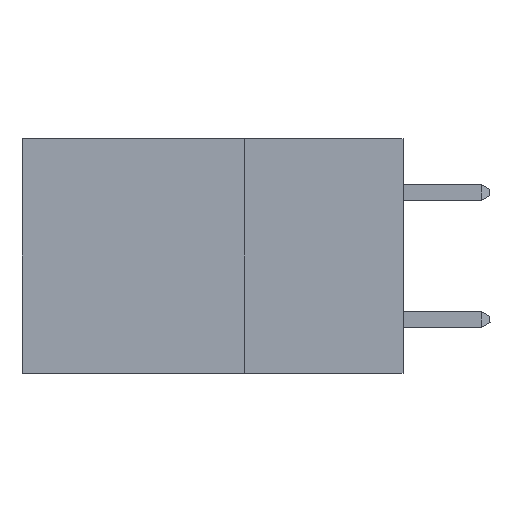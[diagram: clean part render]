
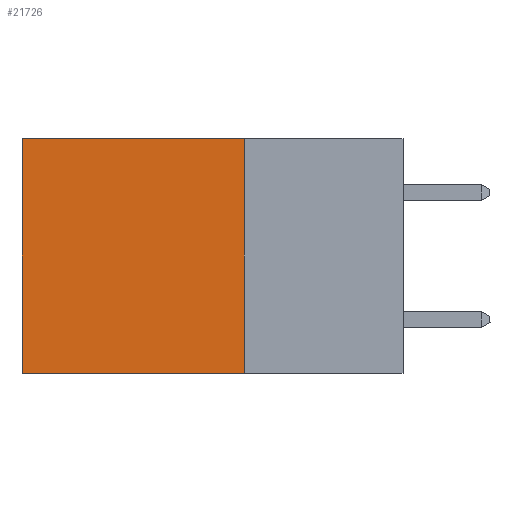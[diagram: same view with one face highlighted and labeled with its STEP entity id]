
A CAD part, left-side view. The second image highlights one B-rep face of the part: STEP entity #21726.
In plain terms, the highlighted planar face has unit normal (-1, 0, 0).
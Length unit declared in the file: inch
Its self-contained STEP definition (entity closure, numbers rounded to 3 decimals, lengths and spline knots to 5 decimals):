
#52 = PLANE ( 'NONE',  #2230 ) ;
#2230 = AXIS2_PLACEMENT_3D ( 'NONE', #5480, #8136, #5143 ) ;
#2328 = DIRECTION ( 'NONE',  ( 0., 0., -1. ) ) ;
#2880 = VERTEX_POINT ( 'NONE', #23018 ) ;
#3109 = CARTESIAN_POINT ( 'NONE',  ( 0.2875, 0.25, -0.37 ) ) ;
#4250 = EDGE_CURVE ( 'NONE', #25213, #13883, #14950, .T. ) ;
#5143 = DIRECTION ( 'NONE',  ( 0., 0., -1. ) ) ;
#5480 = CARTESIAN_POINT ( 'NONE',  ( 0.2875, 0.25, 0. ) ) ;
#6723 = VECTOR ( 'NONE', #2328, 39.37008 ) ;
#7089 = CARTESIAN_POINT ( 'NONE',  ( 0.2875, 0.6, 0. ) ) ;
#8136 = DIRECTION ( 'NONE',  ( 1., 0., 0. ) ) ;
#8657 = CARTESIAN_POINT ( 'NONE',  ( 0.2875, 0.25, -0.37 ) ) ;
#12999 = LINE ( 'NONE', #7089, #6723 ) ;
#13883 = VERTEX_POINT ( 'NONE', #3109 ) ;
#14950 = LINE ( 'NONE', #15391, #26973 ) ;
#15224 = LINE ( 'NONE', #8657, #28020 ) ;
#15391 = CARTESIAN_POINT ( 'NONE',  ( 0.2875, 0.25, 0. ) ) ;
#15589 = FACE_OUTER_BOUND ( 'NONE', #30320, .T. ) ;
#17934 = DIRECTION ( 'NONE',  ( 0., 0., -1. ) ) ;
#18695 = LINE ( 'NONE', #27584, #28721 ) ;
#19436 = CARTESIAN_POINT ( 'NONE',  ( 0.2875, 0.25, 0. ) ) ;
#21438 = EDGE_CURVE ( 'NONE', #13883, #29288, #15224, .T. ) ;
#21726 = ADVANCED_FACE ( 'NONE', ( #15589 ), #52, .F. ) ;
#22998 = ORIENTED_EDGE ( 'NONE', *, *, #4250, .F. ) ;
#23018 = CARTESIAN_POINT ( 'NONE',  ( 0.2875, 0.6, 0. ) ) ;
#23394 = EDGE_CURVE ( 'NONE', #25213, #2880, #18695, .T. ) ;
#25198 = CARTESIAN_POINT ( 'NONE',  ( 0.2875, 0.6, -0.37 ) ) ;
#25213 = VERTEX_POINT ( 'NONE', #19436 ) ;
#26522 = DIRECTION ( 'NONE',  ( 0., 1., 0. ) ) ;
#26973 = VECTOR ( 'NONE', #17934, 39.37008 ) ;
#27584 = CARTESIAN_POINT ( 'NONE',  ( 0.2875, 0.25, 0. ) ) ;
#28020 = VECTOR ( 'NONE', #26522, 39.37008 ) ;
#28215 = ORIENTED_EDGE ( 'NONE', *, *, #23394, .T. ) ;
#28281 = EDGE_CURVE ( 'NONE', #2880, #29288, #12999, .T. ) ;
#28526 = ORIENTED_EDGE ( 'NONE', *, *, #21438, .F. ) ;
#28721 = VECTOR ( 'NONE', #32722, 39.37008 ) ;
#29288 = VERTEX_POINT ( 'NONE', #25198 ) ;
#30320 = EDGE_LOOP ( 'NONE', ( #30427, #28526, #22998, #28215 ) ) ;
#30427 = ORIENTED_EDGE ( 'NONE', *, *, #28281, .T. ) ;
#32722 = DIRECTION ( 'NONE',  ( 0., 1., 0. ) ) ;
